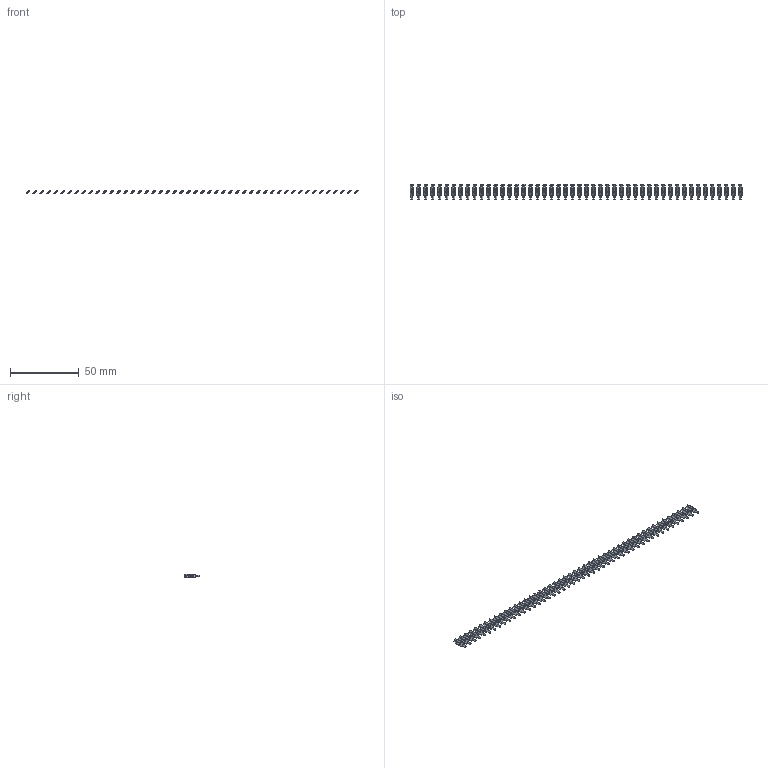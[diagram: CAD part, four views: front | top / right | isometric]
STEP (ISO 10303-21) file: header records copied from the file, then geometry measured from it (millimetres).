
FILE_DESCRIPTION (( 'STEP AP203' ), '1' );
FILE_NAME ('106-048-250-200.STEP', '2020-04-16T20:27:46', ( '' ), ( '' ), 'SwSTEP 2.0', 'SolidWorks 2016', '' );
FILE_SCHEMA (( 'CONFIG_CONTROL_DESIGN' ));
Length unit declared in the file: inch
Products named in the file (2): 106-048-250-200; 100-290-001_100-290-250
Assembly tree (48 placements, depth 2):
  106-048-250-200
    100-290-001_100-290-250  x48
Bounding box: 241.29 x 11.48 x 2.53 mm (x, y, z)
Volume: 749 mm3; surface area: 3520.8 mm2
Topology: 48 solids, 48 shells, 1152 faces, 3168 edges, 2112 vertices
Faces by surface type: plane 960, cylinder 192
Entity records: 2462 total; most frequent: DIRECTION 220, CARTESIAN_POINT 197, ORIENTED_EDGE 132, COORDINATED_UNIVERSAL_TIME_OFFSET 106, CALENDAR_DATE 106, LOCAL_TIME 106, DATE_AND_TIME 106, AXIS2_PLACEMENT_3D 83
